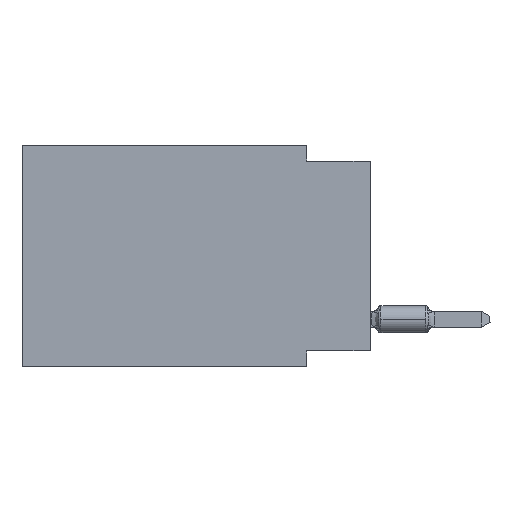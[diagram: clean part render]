
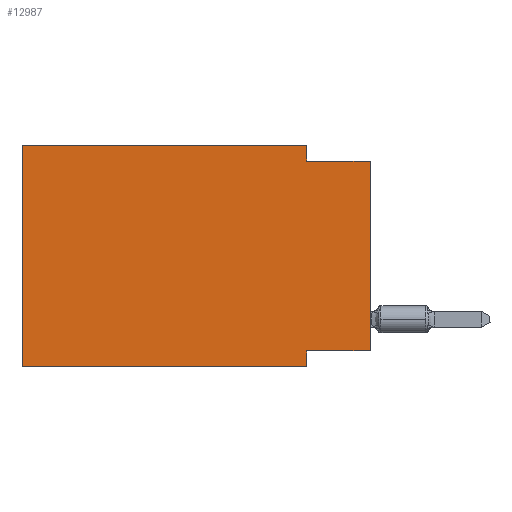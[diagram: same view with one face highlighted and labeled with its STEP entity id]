
A CAD part, left-side view. The second image highlights one B-rep face of the part: STEP entity #12987.
In plain terms, the highlighted planar face has unit normal (-1, 0, 0).
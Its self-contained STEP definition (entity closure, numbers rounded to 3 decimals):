
#3601 = CARTESIAN_POINT ( 'NONE',  ( 0., 0., -0.635 ) ) ;
#3674 = DIRECTION ( 'NONE',  ( 1., 0., 0. ) ) ;
#4515 = FACE_OUTER_BOUND ( 'NONE', #28069, .T. ) ;
#6901 = DIRECTION ( 'NONE',  ( 0., -1., 0. ) ) ;
#7517 = ORIENTED_EDGE ( 'NONE', *, *, #37526, .F. ) ;
#10017 = VECTOR ( 'NONE', #52833, 1000. ) ;
#10378 = EDGE_CURVE ( 'NONE', #31063, #21513, #14667, .T. ) ;
#11626 = EDGE_CURVE ( 'NONE', #22584, #29700, #19826, .T. ) ;
#11935 = DIRECTION ( 'NONE',  ( 0., -1., 0. ) ) ;
#12302 = PLANE ( 'NONE',  #17183 ) ;
#12987 = ADVANCED_FACE ( 'NONE', ( #4515 ), #12302, .F. ) ;
#13055 = VECTOR ( 'NONE', #33305, 1000. ) ;
#14667 = LINE ( 'NONE', #20097, #13055 ) ;
#16035 = CARTESIAN_POINT ( 'NONE',  ( 0., 2.54, -8.255 ) ) ;
#17183 = AXIS2_PLACEMENT_3D ( 'NONE', #34954, #3674, #21472 ) ;
#17344 = EDGE_CURVE ( 'NONE', #25397, #29700, #48572, .T. ) ;
#17835 = LINE ( 'NONE', #35335, #10017 ) ;
#18027 = CARTESIAN_POINT ( 'NONE',  ( 0., 13.97, 0. ) ) ;
#19826 = LINE ( 'NONE', #54834, #39221 ) ;
#20097 = CARTESIAN_POINT ( 'NONE',  ( 0., 0., -0.635 ) ) ;
#21386 = CARTESIAN_POINT ( 'NONE',  ( 0., 2.54, -8.89 ) ) ;
#21453 = CARTESIAN_POINT ( 'NONE',  ( 0., 2.54, -0.635 ) ) ;
#21472 = DIRECTION ( 'NONE',  ( 0., 0., -1. ) ) ;
#21513 = VERTEX_POINT ( 'NONE', #3601 ) ;
#21697 = ORIENTED_EDGE ( 'NONE', *, *, #36292, .T. ) ;
#22584 = VERTEX_POINT ( 'NONE', #41027 ) ;
#24272 = DIRECTION ( 'NONE',  ( 0., 0., 1. ) ) ;
#25397 = VERTEX_POINT ( 'NONE', #16035 ) ;
#28069 = EDGE_LOOP ( 'NONE', ( #21697, #45922, #35888, #7517, #31497, #28201, #41209, #45010 ) ) ;
#28201 = ORIENTED_EDGE ( 'NONE', *, *, #11626, .T. ) ;
#29154 = LINE ( 'NONE', #46942, #32637 ) ;
#29700 = VERTEX_POINT ( 'NONE', #21386 ) ;
#29916 = LINE ( 'NONE', #33657, #44851 ) ;
#30116 = EDGE_CURVE ( 'NONE', #35863, #31063, #29916, .T. ) ;
#30333 = EDGE_CURVE ( 'NONE', #52888, #25397, #17835, .T. ) ;
#31063 = VERTEX_POINT ( 'NONE', #21453 ) ;
#31497 = ORIENTED_EDGE ( 'NONE', *, *, #40898, .F. ) ;
#31991 = VERTEX_POINT ( 'NONE', #18027 ) ;
#32637 = VECTOR ( 'NONE', #11935, 1000. ) ;
#33032 = CARTESIAN_POINT ( 'NONE',  ( 0., 13.97, 0. ) ) ;
#33305 = DIRECTION ( 'NONE',  ( 0., -1., 0. ) ) ;
#33657 = CARTESIAN_POINT ( 'NONE',  ( 0., 2.54, 0. ) ) ;
#33724 = CARTESIAN_POINT ( 'NONE',  ( 0., 0., 0. ) ) ;
#34954 = CARTESIAN_POINT ( 'NONE',  ( 0., 13.97, 0. ) ) ;
#35335 = CARTESIAN_POINT ( 'NONE',  ( 0., 0., -8.255 ) ) ;
#35863 = VERTEX_POINT ( 'NONE', #38095 ) ;
#35888 = ORIENTED_EDGE ( 'NONE', *, *, #30116, .F. ) ;
#36001 = CARTESIAN_POINT ( 'NONE',  ( 0., 0., -8.255 ) ) ;
#36292 = EDGE_CURVE ( 'NONE', #52888, #21513, #42355, .T. ) ;
#37526 = EDGE_CURVE ( 'NONE', #31991, #35863, #29154, .T. ) ;
#38095 = CARTESIAN_POINT ( 'NONE',  ( 0., 2.54, 0. ) ) ;
#38187 = DIRECTION ( 'NONE',  ( 0., 0., 1. ) ) ;
#39221 = VECTOR ( 'NONE', #6901, 1000. ) ;
#40898 = EDGE_CURVE ( 'NONE', #22584, #31991, #41921, .T. ) ;
#41027 = CARTESIAN_POINT ( 'NONE',  ( 0., 13.97, -8.89 ) ) ;
#41209 = ORIENTED_EDGE ( 'NONE', *, *, #17344, .F. ) ;
#41921 = LINE ( 'NONE', #33032, #43844 ) ;
#42355 = LINE ( 'NONE', #33724, #46836 ) ;
#43844 = VECTOR ( 'NONE', #38187, 1000. ) ;
#44851 = VECTOR ( 'NONE', #47418, 1000. ) ;
#45010 = ORIENTED_EDGE ( 'NONE', *, *, #30333, .F. ) ;
#45414 = DIRECTION ( 'NONE',  ( 0., 0., -1. ) ) ;
#45922 = ORIENTED_EDGE ( 'NONE', *, *, #10378, .F. ) ;
#46836 = VECTOR ( 'NONE', #24272, 1000. ) ;
#46942 = CARTESIAN_POINT ( 'NONE',  ( 0., 13.97, 0. ) ) ;
#47418 = DIRECTION ( 'NONE',  ( 0., 0., -1. ) ) ;
#48572 = LINE ( 'NONE', #53161, #55977 ) ;
#52833 = DIRECTION ( 'NONE',  ( 0., 1., 0. ) ) ;
#52888 = VERTEX_POINT ( 'NONE', #36001 ) ;
#53161 = CARTESIAN_POINT ( 'NONE',  ( 0., 2.54, -8.89 ) ) ;
#54834 = CARTESIAN_POINT ( 'NONE',  ( 0., 13.97, -8.89 ) ) ;
#55977 = VECTOR ( 'NONE', #45414, 1000. ) ;
